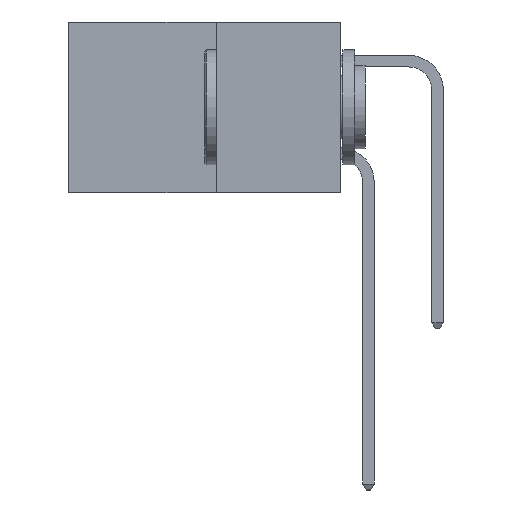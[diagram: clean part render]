
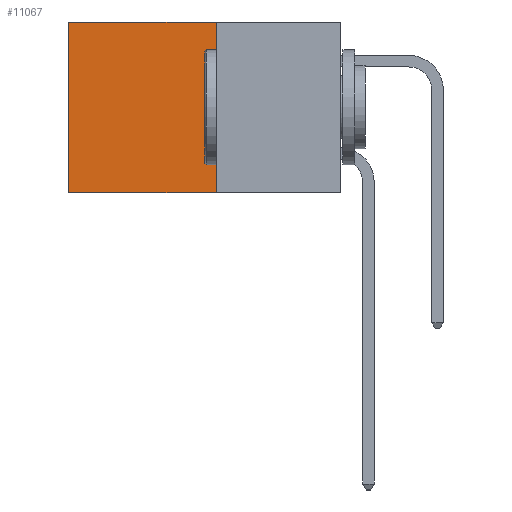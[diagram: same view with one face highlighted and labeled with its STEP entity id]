
A CAD part, left-side view. The second image highlights one B-rep face of the part: STEP entity #11067.
In plain terms, the highlighted planar face has unit normal (-1, 0, 0).
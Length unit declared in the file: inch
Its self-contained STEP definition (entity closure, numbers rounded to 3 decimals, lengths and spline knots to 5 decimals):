
#49 = LINE ( 'NONE', #11064, #9613 ) ;
#214 = LINE ( 'NONE', #11673, #495 ) ;
#267 = EDGE_CURVE ( 'NONE', #1427, #6630, #4707, .T. ) ;
#464 = CARTESIAN_POINT ( 'NONE',  ( 0.277, 0.59, 0. ) ) ;
#495 = VECTOR ( 'NONE', #10993, 39.37008 ) ;
#1037 = EDGE_CURVE ( 'NONE', #11035, #7089, #10495, .T. ) ;
#1352 = CARTESIAN_POINT ( 'NONE',  ( 0.277, 0.59, -0.37 ) ) ;
#1427 = VERTEX_POINT ( 'NONE', #464 ) ;
#1607 = DIRECTION ( 'NONE',  ( 0., 0., -1. ) ) ;
#1935 = DIRECTION ( 'NONE',  ( 0., 0., -1. ) ) ;
#2247 = EDGE_CURVE ( 'NONE', #11035, #1427, #214, .T. ) ;
#2522 = EDGE_CURVE ( 'NONE', #7089, #6630, #49, .T. ) ;
#2839 = AXIS2_PLACEMENT_3D ( 'NONE', #7137, #7168, #1607 ) ;
#4227 = ORIENTED_EDGE ( 'NONE', *, *, #2247, .T. ) ;
#4707 = LINE ( 'NONE', #7273, #6613 ) ;
#5080 = ORIENTED_EDGE ( 'NONE', *, *, #1037, .F. ) ;
#5196 = CARTESIAN_POINT ( 'NONE',  ( 0.277, 0.27, -0.37 ) ) ;
#5813 = ORIENTED_EDGE ( 'NONE', *, *, #2522, .F. ) ;
#6008 = EDGE_LOOP ( 'NONE', ( #6058, #5813, #5080, #4227 ) ) ;
#6058 = ORIENTED_EDGE ( 'NONE', *, *, #267, .T. ) ;
#6223 = CARTESIAN_POINT ( 'NONE',  ( 0.277, 0.27, -0.37 ) ) ;
#6613 = VECTOR ( 'NONE', #1935, 39.37008 ) ;
#6630 = VERTEX_POINT ( 'NONE', #1352 ) ;
#7089 = VERTEX_POINT ( 'NONE', #6223 ) ;
#7137 = CARTESIAN_POINT ( 'NONE',  ( 0.277, 0.27, -0.37 ) ) ;
#7168 = DIRECTION ( 'NONE',  ( 1., 0., 0. ) ) ;
#7273 = CARTESIAN_POINT ( 'NONE',  ( 0.277, 0.59, -0.37 ) ) ;
#7474 = FACE_OUTER_BOUND ( 'NONE', #6008, .T. ) ;
#8062 = VECTOR ( 'NONE', #11617, 39.37008 ) ;
#9613 = VECTOR ( 'NONE', #11566, 39.37008 ) ;
#10495 = LINE ( 'NONE', #5196, #8062 ) ;
#10805 = CARTESIAN_POINT ( 'NONE',  ( 0.277, 0.27, 0. ) ) ;
#10843 = PLANE ( 'NONE',  #2839 ) ;
#10993 = DIRECTION ( 'NONE',  ( 0., 1., 0. ) ) ;
#11035 = VERTEX_POINT ( 'NONE', #10805 ) ;
#11064 = CARTESIAN_POINT ( 'NONE',  ( 0.277, 0.27, -0.37 ) ) ;
#11067 = ADVANCED_FACE ( 'NONE', ( #7474 ), #10843, .F. ) ;
#11566 = DIRECTION ( 'NONE',  ( 0., 1., 0. ) ) ;
#11617 = DIRECTION ( 'NONE',  ( 0., 0., -1. ) ) ;
#11673 = CARTESIAN_POINT ( 'NONE',  ( 0.277, 0.27, 0. ) ) ;
